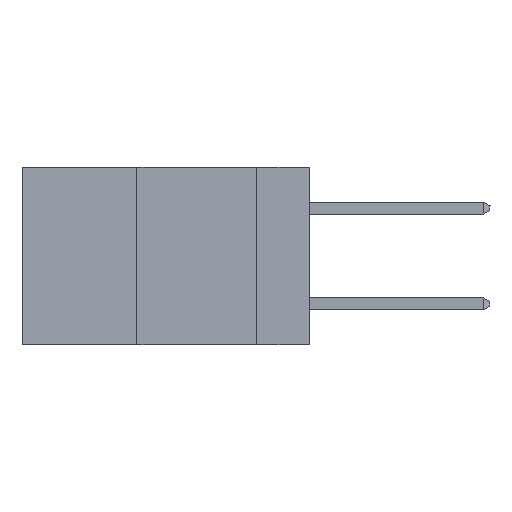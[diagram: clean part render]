
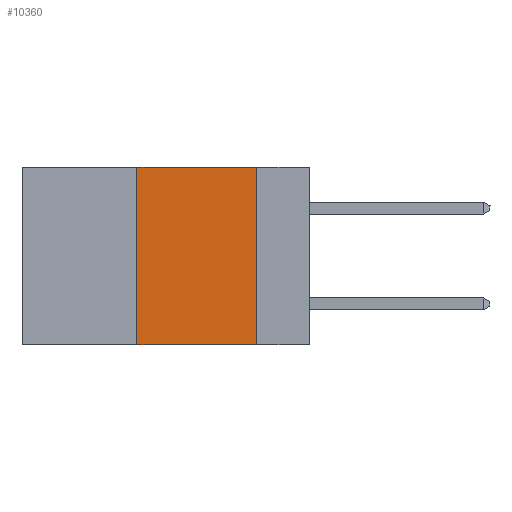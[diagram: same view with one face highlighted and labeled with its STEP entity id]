
A CAD part, left-side view. The second image highlights one B-rep face of the part: STEP entity #10360.
In plain terms, the highlighted planar face has unit normal (-1, 0, 0).
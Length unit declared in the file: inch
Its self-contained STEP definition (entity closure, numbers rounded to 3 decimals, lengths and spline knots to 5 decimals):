
#127 = VERTEX_POINT ( 'NONE', #1798 ) ;
#363 = PLANE ( 'NONE',  #7875 ) ;
#541 = LINE ( 'NONE', #10837, #8239 ) ;
#1169 = VECTOR ( 'NONE', #5381, 39.37008 ) ;
#1324 = DIRECTION ( 'NONE',  ( 0., 0., -1. ) ) ;
#1798 = CARTESIAN_POINT ( 'NONE',  ( 0., 0.11, 0. ) ) ;
#1835 = VERTEX_POINT ( 'NONE', #3248 ) ;
#2060 = DIRECTION ( 'NONE',  ( 1., 0., 0. ) ) ;
#2251 = CARTESIAN_POINT ( 'NONE',  ( 0., 0.36, -0.37 ) ) ;
#2328 = EDGE_CURVE ( 'NONE', #7374, #1835, #10644, .T. ) ;
#3025 = ORIENTED_EDGE ( 'NONE', *, *, #2328, .F. ) ;
#3103 = VECTOR ( 'NONE', #4016, 39.37008 ) ;
#3248 = CARTESIAN_POINT ( 'NONE',  ( 0., 0.36, 0. ) ) ;
#3555 = EDGE_CURVE ( 'NONE', #7374, #7293, #541, .T. ) ;
#4016 = DIRECTION ( 'NONE',  ( 0., 0., -1. ) ) ;
#4094 = CARTESIAN_POINT ( 'NONE',  ( 0., 0.11, 0. ) ) ;
#4417 = EDGE_LOOP ( 'NONE', ( #8607, #9666, #3025, #10889 ) ) ;
#5381 = DIRECTION ( 'NONE',  ( 0., -1., 0. ) ) ;
#5534 = CARTESIAN_POINT ( 'NONE',  ( 0., 0.6, 0. ) ) ;
#5977 = LINE ( 'NONE', #9561, #1169 ) ;
#6709 = EDGE_CURVE ( 'NONE', #127, #7293, #7896, .T. ) ;
#6799 = VECTOR ( 'NONE', #7328, 39.37008 ) ;
#7293 = VERTEX_POINT ( 'NONE', #9053 ) ;
#7312 = DIRECTION ( 'NONE',  ( 0., -1., 0. ) ) ;
#7328 = DIRECTION ( 'NONE',  ( 0., 0., 1. ) ) ;
#7374 = VERTEX_POINT ( 'NONE', #2251 ) ;
#7856 = EDGE_CURVE ( 'NONE', #1835, #127, #5977, .T. ) ;
#7875 = AXIS2_PLACEMENT_3D ( 'NONE', #5534, #2060, #1324 ) ;
#7896 = LINE ( 'NONE', #4094, #3103 ) ;
#8169 = FACE_OUTER_BOUND ( 'NONE', #4417, .T. ) ;
#8229 = CARTESIAN_POINT ( 'NONE',  ( 0., 0.36, 0. ) ) ;
#8239 = VECTOR ( 'NONE', #7312, 39.37008 ) ;
#8607 = ORIENTED_EDGE ( 'NONE', *, *, #6709, .F. ) ;
#9053 = CARTESIAN_POINT ( 'NONE',  ( 0., 0.11, -0.37 ) ) ;
#9561 = CARTESIAN_POINT ( 'NONE',  ( 0., 0.6, 0. ) ) ;
#9666 = ORIENTED_EDGE ( 'NONE', *, *, #7856, .F. ) ;
#10360 = ADVANCED_FACE ( 'NONE', ( #8169 ), #363, .F. ) ;
#10644 = LINE ( 'NONE', #8229, #6799 ) ;
#10837 = CARTESIAN_POINT ( 'NONE',  ( 0., 0.6, -0.37 ) ) ;
#10889 = ORIENTED_EDGE ( 'NONE', *, *, #3555, .T. ) ;
